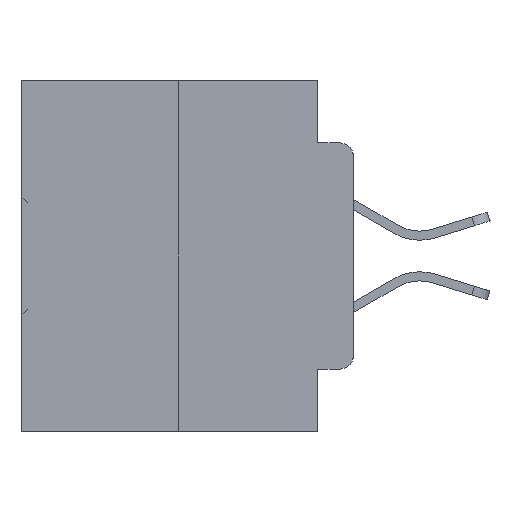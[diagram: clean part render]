
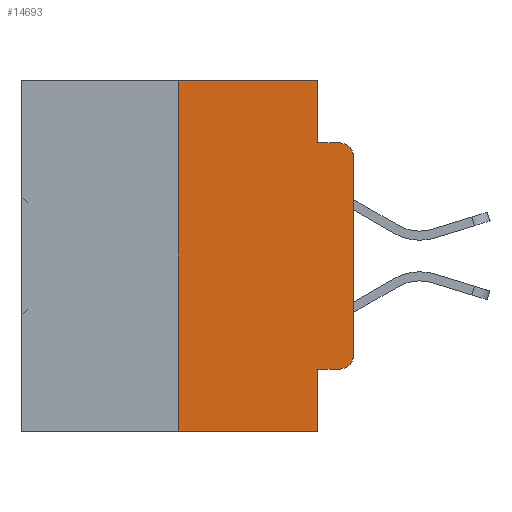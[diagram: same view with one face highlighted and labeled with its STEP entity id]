
A CAD part, left-side view. The second image highlights one B-rep face of the part: STEP entity #14693.
In plain terms, the highlighted planar face has unit normal (-1, 0, 0).
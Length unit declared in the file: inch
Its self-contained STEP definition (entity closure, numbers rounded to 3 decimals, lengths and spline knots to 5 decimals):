
#539 = CARTESIAN_POINT ( 'NONE',  ( 0., 0.051, -0.4115 ) ) ;
#759 = VERTEX_POINT ( 'NONE', #3875 ) ;
#2090 = VERTEX_POINT ( 'NONE', #19464 ) ;
#3153 = CARTESIAN_POINT ( 'NONE',  ( 0., 0.473, -0.5 ) ) ;
#3307 = VERTEX_POINT ( 'NONE', #4451 ) ;
#3319 = EDGE_CURVE ( 'NONE', #17361, #10973, #13338, .T. ) ;
#3543 = CARTESIAN_POINT ( 'NONE',  ( 0., 0.051, -0.4115 ) ) ;
#3783 = CARTESIAN_POINT ( 'NONE',  ( 0., 0., 0. ) ) ;
#3875 = CARTESIAN_POINT ( 'NONE',  ( 0., 0.02, -0.4115 ) ) ;
#3924 = CARTESIAN_POINT ( 'NONE',  ( 0., 0.051, 0. ) ) ;
#4451 = CARTESIAN_POINT ( 'NONE',  ( 0., 0.02, -0.0885 ) ) ;
#4853 = EDGE_CURVE ( 'NONE', #23029, #3307, #6883, .T. ) ;
#5592 = EDGE_CURVE ( 'NONE', #33158, #15901, #11126, .T. ) ;
#5751 = DIRECTION ( 'NONE',  ( -1., 0., 0. ) ) ;
#6289 = DIRECTION ( 'NONE',  ( 0., -1., 0. ) ) ;
#6414 = FACE_OUTER_BOUND ( 'NONE', #24344, .T. ) ;
#6611 = EDGE_CURVE ( 'NONE', #30073, #18128, #29755, .T. ) ;
#6883 = LINE ( 'NONE', #29570, #21201 ) ;
#7237 = CARTESIAN_POINT ( 'NONE',  ( 0., 0.051, 0. ) ) ;
#7810 = DIRECTION ( 'NONE',  ( 0., -1., 0. ) ) ;
#8199 = VECTOR ( 'NONE', #30007, 39.37008 ) ;
#8619 = DIRECTION ( 'NONE',  ( 1., 0., 0. ) ) ;
#8704 = DIRECTION ( 'NONE',  ( 0., -1., 0. ) ) ;
#9233 = DIRECTION ( 'NONE',  ( 0., 0., 1. ) ) ;
#9761 = LINE ( 'NONE', #3153, #23134 ) ;
#10582 = CARTESIAN_POINT ( 'NONE',  ( 0., 0.473, 0. ) ) ;
#10839 = ORIENTED_EDGE ( 'NONE', *, *, #28228, .T. ) ;
#10973 = VERTEX_POINT ( 'NONE', #27853 ) ;
#11126 = LINE ( 'NONE', #3783, #26925 ) ;
#11237 = CARTESIAN_POINT ( 'NONE',  ( 0., 0.25, 0. ) ) ;
#11436 = CARTESIAN_POINT ( 'NONE',  ( 0., 0.25, 0. ) ) ;
#13338 = LINE ( 'NONE', #7237, #18759 ) ;
#13680 = DIRECTION ( 'NONE',  ( 0., -1., 0. ) ) ;
#13772 = ORIENTED_EDGE ( 'NONE', *, *, #32643, .F. ) ;
#14422 = CARTESIAN_POINT ( 'NONE',  ( 0., 0.02, -0.1085 ) ) ;
#14693 = ADVANCED_FACE ( 'NONE', ( #6414 ), #24638, .F. ) ;
#15440 = DIRECTION ( 'NONE',  ( 0., 0., -1. ) ) ;
#15901 = VERTEX_POINT ( 'NONE', #26961 ) ;
#16525 = VECTOR ( 'NONE', #7810, 39.37008 ) ;
#16698 = EDGE_CURVE ( 'NONE', #17361, #759, #33697, .T. ) ;
#17104 = DIRECTION ( 'NONE',  ( 0., 0., -1. ) ) ;
#17326 = EDGE_CURVE ( 'NONE', #2090, #30073, #22469, .T. ) ;
#17361 = VERTEX_POINT ( 'NONE', #539 ) ;
#17545 = ORIENTED_EDGE ( 'NONE', *, *, #17326, .F. ) ;
#18128 = VERTEX_POINT ( 'NONE', #3924 ) ;
#18759 = VECTOR ( 'NONE', #15440, 39.37008 ) ;
#19296 = CARTESIAN_POINT ( 'NONE',  ( 0., 0.473, 0. ) ) ;
#19395 = DIRECTION ( 'NONE',  ( 0., 0., -1. ) ) ;
#19464 = CARTESIAN_POINT ( 'NONE',  ( 0., 0.25, -0.5 ) ) ;
#19596 = VECTOR ( 'NONE', #6289, 39.37008 ) ;
#19897 = AXIS2_PLACEMENT_3D ( 'NONE', #14422, #32950, #17104 ) ;
#20780 = CIRCLE ( 'NONE', #27544, 0.02 ) ;
#21201 = VECTOR ( 'NONE', #13680, 39.37008 ) ;
#21922 = CARTESIAN_POINT ( 'NONE',  ( 0., 0.02, -0.3915 ) ) ;
#22049 = ORIENTED_EDGE ( 'NONE', *, *, #33295, .T. ) ;
#22469 = LINE ( 'NONE', #11436, #8199 ) ;
#22525 = ORIENTED_EDGE ( 'NONE', *, *, #4853, .F. ) ;
#23029 = VERTEX_POINT ( 'NONE', #32670 ) ;
#23134 = VECTOR ( 'NONE', #8704, 39.37008 ) ;
#24344 = EDGE_LOOP ( 'NONE', ( #32856, #10839, #22525, #13772, #25394, #17545, #27007, #32387, #30748, #22049 ) ) ;
#24578 = DIRECTION ( 'NONE',  ( 0., 0., -1. ) ) ;
#24638 = PLANE ( 'NONE',  #27781 ) ;
#25394 = ORIENTED_EDGE ( 'NONE', *, *, #6611, .F. ) ;
#25773 = VECTOR ( 'NONE', #19395, 39.37008 ) ;
#26450 = CIRCLE ( 'NONE', #19897, 0.02 ) ;
#26524 = CARTESIAN_POINT ( 'NONE',  ( 0., 0., -0.3915 ) ) ;
#26925 = VECTOR ( 'NONE', #9233, 39.37008 ) ;
#26961 = CARTESIAN_POINT ( 'NONE',  ( 0., 0., -0.1085 ) ) ;
#27007 = ORIENTED_EDGE ( 'NONE', *, *, #28794, .T. ) ;
#27271 = DIRECTION ( 'NONE',  ( 0., 0., -1. ) ) ;
#27544 = AXIS2_PLACEMENT_3D ( 'NONE', #21922, #5751, #24578 ) ;
#27781 = AXIS2_PLACEMENT_3D ( 'NONE', #19296, #8619, #27271 ) ;
#27853 = CARTESIAN_POINT ( 'NONE',  ( 0., 0.051, -0.5 ) ) ;
#28228 = EDGE_CURVE ( 'NONE', #15901, #3307, #26450, .T. ) ;
#28794 = EDGE_CURVE ( 'NONE', #2090, #10973, #9761, .T. ) ;
#29570 = CARTESIAN_POINT ( 'NONE',  ( 0., 0.051, -0.0885 ) ) ;
#29755 = LINE ( 'NONE', #10582, #16525 ) ;
#30007 = DIRECTION ( 'NONE',  ( 0., 0., 1. ) ) ;
#30073 = VERTEX_POINT ( 'NONE', #11237 ) ;
#30748 = ORIENTED_EDGE ( 'NONE', *, *, #16698, .T. ) ;
#32387 = ORIENTED_EDGE ( 'NONE', *, *, #3319, .F. ) ;
#32581 = CARTESIAN_POINT ( 'NONE',  ( 0., 0.051, 0. ) ) ;
#32643 = EDGE_CURVE ( 'NONE', #18128, #23029, #32814, .T. ) ;
#32670 = CARTESIAN_POINT ( 'NONE',  ( 0., 0.051, -0.0885 ) ) ;
#32814 = LINE ( 'NONE', #32581, #25773 ) ;
#32856 = ORIENTED_EDGE ( 'NONE', *, *, #5592, .T. ) ;
#32950 = DIRECTION ( 'NONE',  ( -1., 0., 0. ) ) ;
#33158 = VERTEX_POINT ( 'NONE', #26524 ) ;
#33295 = EDGE_CURVE ( 'NONE', #759, #33158, #20780, .T. ) ;
#33697 = LINE ( 'NONE', #3543, #19596 ) ;
